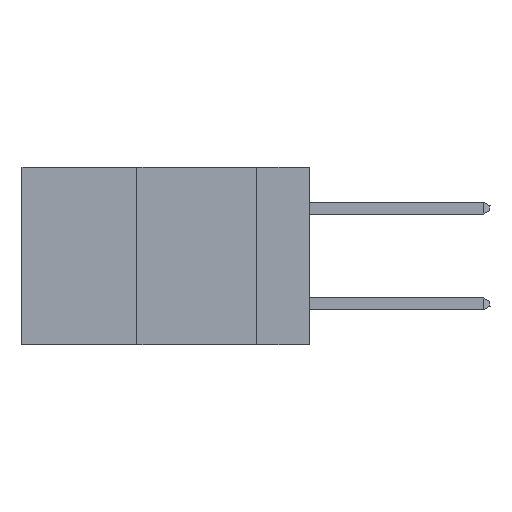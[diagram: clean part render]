
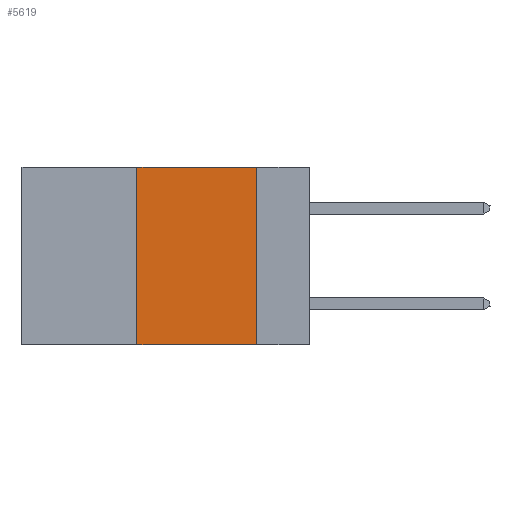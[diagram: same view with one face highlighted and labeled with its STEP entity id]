
A CAD part, left-side view. The second image highlights one B-rep face of the part: STEP entity #5619.
In plain terms, the highlighted planar face has unit normal (-1, 0, 0).
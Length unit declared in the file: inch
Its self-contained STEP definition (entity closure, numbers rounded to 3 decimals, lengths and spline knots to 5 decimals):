
#741 = DIRECTION ( 'NONE',  ( 1., 0., 0. ) ) ;
#1145 = ORIENTED_EDGE ( 'NONE', *, *, #32041, .F. ) ;
#2792 = VERTEX_POINT ( 'NONE', #22623 ) ;
#3848 = VERTEX_POINT ( 'NONE', #23249 ) ;
#4810 = FACE_OUTER_BOUND ( 'NONE', #39656, .T. ) ;
#4891 = CARTESIAN_POINT ( 'NONE',  ( 0., 0.6, 0. ) ) ;
#5619 = ADVANCED_FACE ( 'NONE', ( #4810 ), #10669, .F. ) ;
#6817 = CARTESIAN_POINT ( 'NONE',  ( 0., 0.36, 0. ) ) ;
#8775 = EDGE_CURVE ( 'NONE', #12313, #3848, #23303, .T. ) ;
#9584 = LINE ( 'NONE', #17868, #25686 ) ;
#10641 = CARTESIAN_POINT ( 'NONE',  ( 0., 0.36, 0. ) ) ;
#10669 = PLANE ( 'NONE',  #20064 ) ;
#11262 = VECTOR ( 'NONE', #30933, 39.37008 ) ;
#11853 = VERTEX_POINT ( 'NONE', #24084 ) ;
#12313 = VERTEX_POINT ( 'NONE', #6817 ) ;
#13231 = EDGE_CURVE ( 'NONE', #2792, #11853, #36698, .T. ) ;
#16577 = LINE ( 'NONE', #10641, #24155 ) ;
#17111 = DIRECTION ( 'NONE',  ( 0., 0., -1. ) ) ;
#17868 = CARTESIAN_POINT ( 'NONE',  ( 0., 0.11, 0. ) ) ;
#20064 = AXIS2_PLACEMENT_3D ( 'NONE', #26567, #741, #17111 ) ;
#20498 = ORIENTED_EDGE ( 'NONE', *, *, #32282, .F. ) ;
#21055 = DIRECTION ( 'NONE',  ( 0., -1., 0. ) ) ;
#22284 = VECTOR ( 'NONE', #21055, 39.37008 ) ;
#22623 = CARTESIAN_POINT ( 'NONE',  ( 0., 0.36, -0.37 ) ) ;
#23249 = CARTESIAN_POINT ( 'NONE',  ( 0., 0.11, 0. ) ) ;
#23303 = LINE ( 'NONE', #4891, #22284 ) ;
#24084 = CARTESIAN_POINT ( 'NONE',  ( 0., 0.11, -0.37 ) ) ;
#24155 = VECTOR ( 'NONE', #36153, 39.37008 ) ;
#25686 = VECTOR ( 'NONE', #37047, 39.37008 ) ;
#26567 = CARTESIAN_POINT ( 'NONE',  ( 0., 0.6, 0. ) ) ;
#27023 = ORIENTED_EDGE ( 'NONE', *, *, #8775, .F. ) ;
#27765 = CARTESIAN_POINT ( 'NONE',  ( 0., 0.6, -0.37 ) ) ;
#29012 = ORIENTED_EDGE ( 'NONE', *, *, #13231, .T. ) ;
#30933 = DIRECTION ( 'NONE',  ( 0., -1., 0. ) ) ;
#32041 = EDGE_CURVE ( 'NONE', #3848, #11853, #9584, .T. ) ;
#32282 = EDGE_CURVE ( 'NONE', #2792, #12313, #16577, .T. ) ;
#36153 = DIRECTION ( 'NONE',  ( 0., 0., 1. ) ) ;
#36698 = LINE ( 'NONE', #27765, #11262 ) ;
#37047 = DIRECTION ( 'NONE',  ( 0., 0., -1. ) ) ;
#39656 = EDGE_LOOP ( 'NONE', ( #1145, #27023, #20498, #29012 ) ) ;
